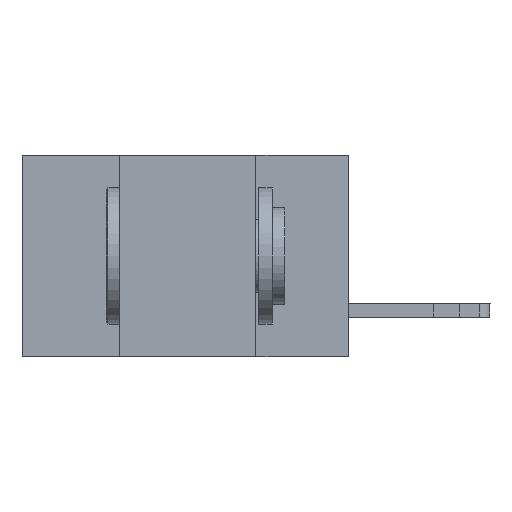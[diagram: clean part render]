
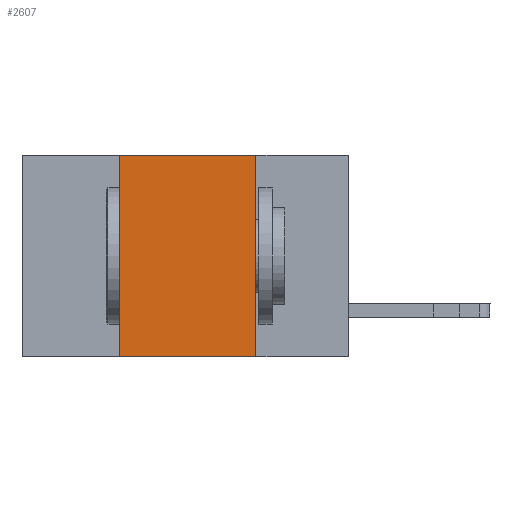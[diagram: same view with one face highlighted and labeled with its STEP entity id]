
A CAD part, left-side view. The second image highlights one B-rep face of the part: STEP entity #2607.
In plain terms, the highlighted planar face has unit normal (-1, 0, 0).
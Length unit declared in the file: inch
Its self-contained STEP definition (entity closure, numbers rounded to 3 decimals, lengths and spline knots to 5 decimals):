
#76 = CARTESIAN_POINT ( 'NONE',  ( 0., 0.6, 0. ) ) ;
#753 = EDGE_CURVE ( 'NONE', #11044, #11104, #833, .T. ) ;
#833 = LINE ( 'NONE', #3474, #10604 ) ;
#894 = ORIENTED_EDGE ( 'NONE', *, *, #2291, .T. ) ;
#1158 = DIRECTION ( 'NONE',  ( 0., 0., -1. ) ) ;
#1214 = EDGE_CURVE ( 'NONE', #3297, #8638, #9561, .T. ) ;
#1228 = CARTESIAN_POINT ( 'NONE',  ( 0., 0.42, 0. ) ) ;
#1309 = FACE_OUTER_BOUND ( 'NONE', #10929, .T. ) ;
#1753 = VECTOR ( 'NONE', #6948, 39.37008 ) ;
#2016 = EDGE_CURVE ( 'NONE', #8638, #11044, #9522, .T. ) ;
#2291 = EDGE_CURVE ( 'NONE', #3297, #11104, #7667, .T. ) ;
#2607 = ADVANCED_FACE ( 'NONE', ( #1309 ), #6597, .F. ) ;
#3297 = VERTEX_POINT ( 'NONE', #7951 ) ;
#3474 = CARTESIAN_POINT ( 'NONE',  ( 0., 0.17, -0.37 ) ) ;
#5167 = VECTOR ( 'NONE', #9524, 39.37008 ) ;
#6518 = AXIS2_PLACEMENT_3D ( 'NONE', #6736, #6583, #6580 ) ;
#6580 = DIRECTION ( 'NONE',  ( 0., 0., -1. ) ) ;
#6583 = DIRECTION ( 'NONE',  ( 1., 0., 0. ) ) ;
#6597 = PLANE ( 'NONE',  #6518 ) ;
#6736 = CARTESIAN_POINT ( 'NONE',  ( 0., 0.6, 0. ) ) ;
#6948 = DIRECTION ( 'NONE',  ( 0., 0., 1. ) ) ;
#7107 = VECTOR ( 'NONE', #12416, 39.37008 ) ;
#7529 = CARTESIAN_POINT ( 'NONE',  ( 0., 0.17, 0. ) ) ;
#7667 = LINE ( 'NONE', #9660, #5167 ) ;
#7951 = CARTESIAN_POINT ( 'NONE',  ( 0., 0.42, -0.37 ) ) ;
#8638 = VERTEX_POINT ( 'NONE', #1228 ) ;
#8957 = CARTESIAN_POINT ( 'NONE',  ( 0., 0.42, -0.37 ) ) ;
#9359 = CARTESIAN_POINT ( 'NONE',  ( 0., 0.17, -0.37 ) ) ;
#9522 = LINE ( 'NONE', #76, #7107 ) ;
#9524 = DIRECTION ( 'NONE',  ( 0., -1., 0. ) ) ;
#9561 = LINE ( 'NONE', #8957, #1753 ) ;
#9660 = CARTESIAN_POINT ( 'NONE',  ( 0., 0.6, -0.37 ) ) ;
#10604 = VECTOR ( 'NONE', #1158, 39.37008 ) ;
#10792 = ORIENTED_EDGE ( 'NONE', *, *, #2016, .F. ) ;
#10929 = EDGE_LOOP ( 'NONE', ( #11570, #10792, #11175, #894 ) ) ;
#11044 = VERTEX_POINT ( 'NONE', #7529 ) ;
#11104 = VERTEX_POINT ( 'NONE', #9359 ) ;
#11175 = ORIENTED_EDGE ( 'NONE', *, *, #1214, .F. ) ;
#11570 = ORIENTED_EDGE ( 'NONE', *, *, #753, .F. ) ;
#12416 = DIRECTION ( 'NONE',  ( 0., -1., 0. ) ) ;
